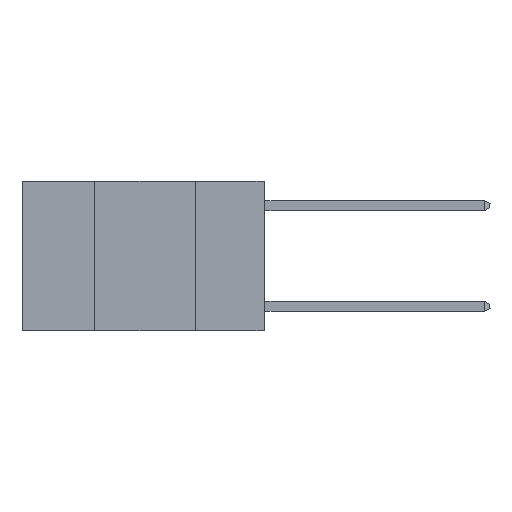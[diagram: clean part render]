
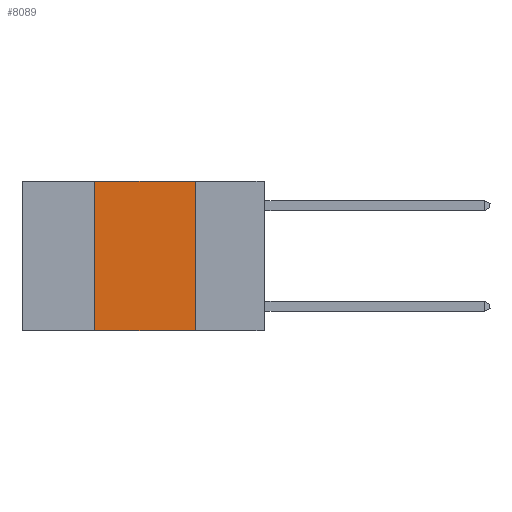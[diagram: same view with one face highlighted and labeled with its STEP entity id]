
A CAD part, left-side view. The second image highlights one B-rep face of the part: STEP entity #8089.
In plain terms, the highlighted planar face has unit normal (-1, 0, 0).
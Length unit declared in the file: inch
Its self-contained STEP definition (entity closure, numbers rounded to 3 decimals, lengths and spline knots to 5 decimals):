
#34 = VERTEX_POINT ( 'NONE', #15011 ) ;
#812 = CARTESIAN_POINT ( 'NONE',  ( 0., 0.42, 0. ) ) ;
#3121 = CARTESIAN_POINT ( 'NONE',  ( 0., 0.6, -0.37 ) ) ;
#3617 = DIRECTION ( 'NONE',  ( 0., 0., -1. ) ) ;
#4224 = EDGE_CURVE ( 'NONE', #34, #7104, #9418, .T. ) ;
#5660 = CARTESIAN_POINT ( 'NONE',  ( 0., 0.6, 0. ) ) ;
#6076 = AXIS2_PLACEMENT_3D ( 'NONE', #5660, #7361, #12211 ) ;
#7104 = VERTEX_POINT ( 'NONE', #11573 ) ;
#7130 = CARTESIAN_POINT ( 'NONE',  ( 0., 0.17, 0. ) ) ;
#7141 = PLANE ( 'NONE',  #6076 ) ;
#7361 = DIRECTION ( 'NONE',  ( 1., 0., 0. ) ) ;
#7894 = CARTESIAN_POINT ( 'NONE',  ( 0., 0.6, 0. ) ) ;
#8089 = ADVANCED_FACE ( 'NONE', ( #8932 ), #7141, .F. ) ;
#8711 = EDGE_CURVE ( 'NONE', #7104, #17670, #16141, .T. ) ;
#8932 = FACE_OUTER_BOUND ( 'NONE', #9203, .T. ) ;
#9203 = EDGE_LOOP ( 'NONE', ( #16925, #14570, #12431, #10809 ) ) ;
#9268 = LINE ( 'NONE', #7130, #20151 ) ;
#9418 = LINE ( 'NONE', #812, #21566 ) ;
#10227 = DIRECTION ( 'NONE',  ( 0., -1., 0. ) ) ;
#10809 = ORIENTED_EDGE ( 'NONE', *, *, #20400, .T. ) ;
#11573 = CARTESIAN_POINT ( 'NONE',  ( 0., 0.42, 0. ) ) ;
#12211 = DIRECTION ( 'NONE',  ( 0., 0., -1. ) ) ;
#12431 = ORIENTED_EDGE ( 'NONE', *, *, #4224, .F. ) ;
#13510 = LINE ( 'NONE', #3121, #18234 ) ;
#14570 = ORIENTED_EDGE ( 'NONE', *, *, #8711, .F. ) ;
#15011 = CARTESIAN_POINT ( 'NONE',  ( 0., 0.42, -0.37 ) ) ;
#16125 = EDGE_CURVE ( 'NONE', #17670, #19026, #9268, .T. ) ;
#16141 = LINE ( 'NONE', #7894, #19804 ) ;
#16925 = ORIENTED_EDGE ( 'NONE', *, *, #16125, .F. ) ;
#17670 = VERTEX_POINT ( 'NONE', #22055 ) ;
#18234 = VECTOR ( 'NONE', #10227, 39.37008 ) ;
#19026 = VERTEX_POINT ( 'NONE', #22160 ) ;
#19423 = DIRECTION ( 'NONE',  ( 0., -1., 0. ) ) ;
#19804 = VECTOR ( 'NONE', #19423, 39.37008 ) ;
#19912 = DIRECTION ( 'NONE',  ( 0., 0., 1. ) ) ;
#20151 = VECTOR ( 'NONE', #3617, 39.37008 ) ;
#20400 = EDGE_CURVE ( 'NONE', #34, #19026, #13510, .T. ) ;
#21566 = VECTOR ( 'NONE', #19912, 39.37008 ) ;
#22055 = CARTESIAN_POINT ( 'NONE',  ( 0., 0.17, 0. ) ) ;
#22160 = CARTESIAN_POINT ( 'NONE',  ( 0., 0.17, -0.37 ) ) ;
